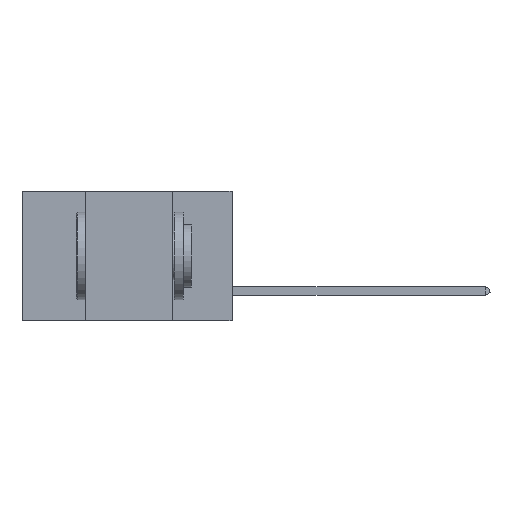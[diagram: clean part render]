
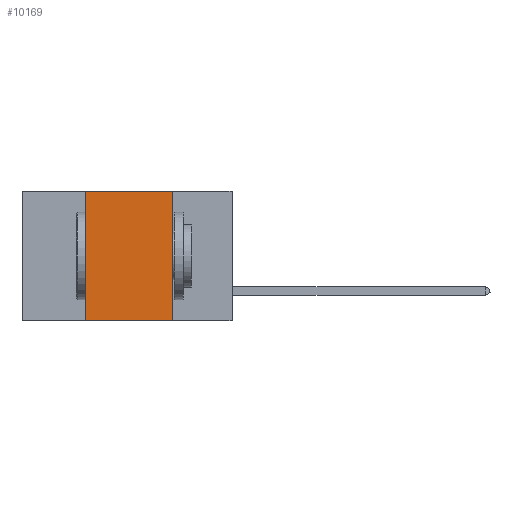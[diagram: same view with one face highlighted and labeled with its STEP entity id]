
A CAD part, left-side view. The second image highlights one B-rep face of the part: STEP entity #10169.
In plain terms, the highlighted planar face has unit normal (-1, 0, 0).
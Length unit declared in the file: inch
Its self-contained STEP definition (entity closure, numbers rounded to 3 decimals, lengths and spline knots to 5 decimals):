
#404 = DIRECTION ( 'NONE',  ( 0., 0., -1. ) ) ;
#987 = AXIS2_PLACEMENT_3D ( 'NONE', #10672, #5136, #404 ) ;
#1065 = LINE ( 'NONE', #13159, #5086 ) ;
#1220 = CARTESIAN_POINT ( 'NONE',  ( 0., 0.17, 0. ) ) ;
#1343 = VECTOR ( 'NONE', #2464, 39.37008 ) ;
#1486 = VECTOR ( 'NONE', #10996, 39.37008 ) ;
#1891 = PLANE ( 'NONE',  #987 ) ;
#2464 = DIRECTION ( 'NONE',  ( 0., 0., -1. ) ) ;
#3445 = DIRECTION ( 'NONE',  ( 0., -1., 0. ) ) ;
#3640 = CARTESIAN_POINT ( 'NONE',  ( 0., 0.42, -0.37 ) ) ;
#4193 = VERTEX_POINT ( 'NONE', #3640 ) ;
#4234 = VERTEX_POINT ( 'NONE', #5031 ) ;
#4978 = CARTESIAN_POINT ( 'NONE',  ( 0., 0.17, 0. ) ) ;
#5031 = CARTESIAN_POINT ( 'NONE',  ( 0., 0.42, 0. ) ) ;
#5086 = VECTOR ( 'NONE', #6319, 39.37008 ) ;
#5136 = DIRECTION ( 'NONE',  ( 1., 0., 0. ) ) ;
#5335 = ORIENTED_EDGE ( 'NONE', *, *, #9661, .F. ) ;
#6029 = LINE ( 'NONE', #10377, #8568 ) ;
#6106 = CARTESIAN_POINT ( 'NONE',  ( 0., 0.17, -0.37 ) ) ;
#6145 = VERTEX_POINT ( 'NONE', #6106 ) ;
#6319 = DIRECTION ( 'NONE',  ( 0., -1., 0. ) ) ;
#6581 = LINE ( 'NONE', #7701, #1486 ) ;
#6604 = LINE ( 'NONE', #1220, #1343 ) ;
#7287 = EDGE_CURVE ( 'NONE', #4234, #7762, #6029, .T. ) ;
#7701 = CARTESIAN_POINT ( 'NONE',  ( 0., 0.42, 0. ) ) ;
#7762 = VERTEX_POINT ( 'NONE', #4978 ) ;
#7880 = EDGE_CURVE ( 'NONE', #4193, #6145, #1065, .T. ) ;
#8568 = VECTOR ( 'NONE', #3445, 39.37008 ) ;
#8702 = ORIENTED_EDGE ( 'NONE', *, *, #9184, .F. ) ;
#9133 = FACE_OUTER_BOUND ( 'NONE', #11150, .T. ) ;
#9184 = EDGE_CURVE ( 'NONE', #7762, #6145, #6604, .T. ) ;
#9249 = ORIENTED_EDGE ( 'NONE', *, *, #7287, .F. ) ;
#9661 = EDGE_CURVE ( 'NONE', #4193, #4234, #6581, .T. ) ;
#10169 = ADVANCED_FACE ( 'NONE', ( #9133 ), #1891, .F. ) ;
#10377 = CARTESIAN_POINT ( 'NONE',  ( 0., 0.6, 0. ) ) ;
#10672 = CARTESIAN_POINT ( 'NONE',  ( 0., 0.6, 0. ) ) ;
#10996 = DIRECTION ( 'NONE',  ( 0., 0., 1. ) ) ;
#11150 = EDGE_LOOP ( 'NONE', ( #8702, #9249, #5335, #11211 ) ) ;
#11211 = ORIENTED_EDGE ( 'NONE', *, *, #7880, .T. ) ;
#13159 = CARTESIAN_POINT ( 'NONE',  ( 0., 0.6, -0.37 ) ) ;
